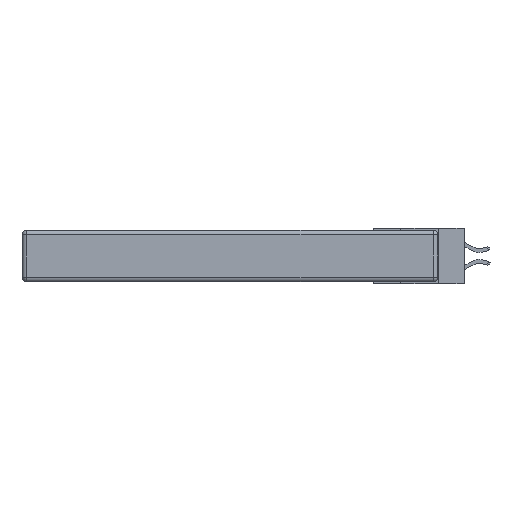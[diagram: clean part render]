
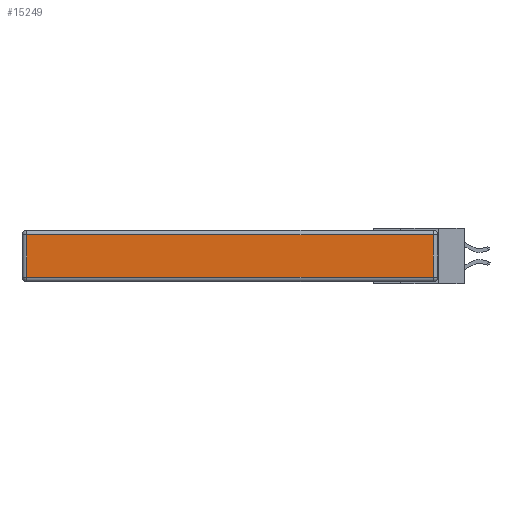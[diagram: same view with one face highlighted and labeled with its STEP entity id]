
A CAD part, left-side view. The second image highlights one B-rep face of the part: STEP entity #15249.
In plain terms, the highlighted planar face has unit normal (-1, 0, 0).
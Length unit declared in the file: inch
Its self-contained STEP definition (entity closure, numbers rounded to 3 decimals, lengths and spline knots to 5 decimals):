
#401 = VERTEX_POINT ( 'NONE', #13322 ) ;
#1496 = VERTEX_POINT ( 'NONE', #17484 ) ;
#3863 = VECTOR ( 'NONE', #16302, 39.37008 ) ;
#3915 = CARTESIAN_POINT ( 'NONE',  ( 0., 0.03, -0.03 ) ) ;
#3958 = EDGE_CURVE ( 'NONE', #401, #19994, #8673, .T. ) ;
#4008 = VECTOR ( 'NONE', #10891, 39.37008 ) ;
#4258 = CARTESIAN_POINT ( 'NONE',  ( 0., 2.72, -0.313 ) ) ;
#8673 = LINE ( 'NONE', #9167, #3863 ) ;
#9167 = CARTESIAN_POINT ( 'NONE',  ( 0., 0.03, -0.343 ) ) ;
#10146 = ORIENTED_EDGE ( 'NONE', *, *, #11585, .T. ) ;
#10213 = VECTOR ( 'NONE', #23134, 39.37008 ) ;
#10362 = CARTESIAN_POINT ( 'NONE',  ( 0., 0., -0.313 ) ) ;
#10759 = EDGE_CURVE ( 'NONE', #19994, #1496, #21318, .T. ) ;
#10891 = DIRECTION ( 'NONE',  ( 0., 1., 0. ) ) ;
#11154 = DIRECTION ( 'NONE',  ( 0., 0., -1. ) ) ;
#11585 = EDGE_CURVE ( 'NONE', #13268, #401, #19304, .T. ) ;
#12382 = ORIENTED_EDGE ( 'NONE', *, *, #14183, .T. ) ;
#13208 = FACE_OUTER_BOUND ( 'NONE', #13372, .T. ) ;
#13268 = VERTEX_POINT ( 'NONE', #4258 ) ;
#13322 = CARTESIAN_POINT ( 'NONE',  ( 0., 0.03, -0.313 ) ) ;
#13372 = EDGE_LOOP ( 'NONE', ( #10146, #13929, #20500, #12382 ) ) ;
#13929 = ORIENTED_EDGE ( 'NONE', *, *, #3958, .T. ) ;
#14183 = EDGE_CURVE ( 'NONE', #1496, #13268, #14924, .T. ) ;
#14343 = PLANE ( 'NONE',  #18110 ) ;
#14815 = CARTESIAN_POINT ( 'NONE',  ( 0., 2.72, -0.343 ) ) ;
#14924 = LINE ( 'NONE', #14815, #21705 ) ;
#15249 = ADVANCED_FACE ( 'NONE', ( #13208 ), #14343, .T. ) ;
#16302 = DIRECTION ( 'NONE',  ( 0., 0., 1. ) ) ;
#17484 = CARTESIAN_POINT ( 'NONE',  ( 0., 2.72, -0.03 ) ) ;
#17973 = CARTESIAN_POINT ( 'NONE',  ( 0., 0., -0.343 ) ) ;
#18110 = AXIS2_PLACEMENT_3D ( 'NONE', #17973, #23156, #23383 ) ;
#19304 = LINE ( 'NONE', #10362, #10213 ) ;
#19994 = VERTEX_POINT ( 'NONE', #3915 ) ;
#20500 = ORIENTED_EDGE ( 'NONE', *, *, #10759, .T. ) ;
#21318 = LINE ( 'NONE', #21779, #4008 ) ;
#21705 = VECTOR ( 'NONE', #11154, 39.37008 ) ;
#21779 = CARTESIAN_POINT ( 'NONE',  ( 0., 2.75, -0.03 ) ) ;
#23134 = DIRECTION ( 'NONE',  ( 0., -1., 0. ) ) ;
#23156 = DIRECTION ( 'NONE',  ( -1., 0., 0. ) ) ;
#23383 = DIRECTION ( 'NONE',  ( 0., 0., 1. ) ) ;
